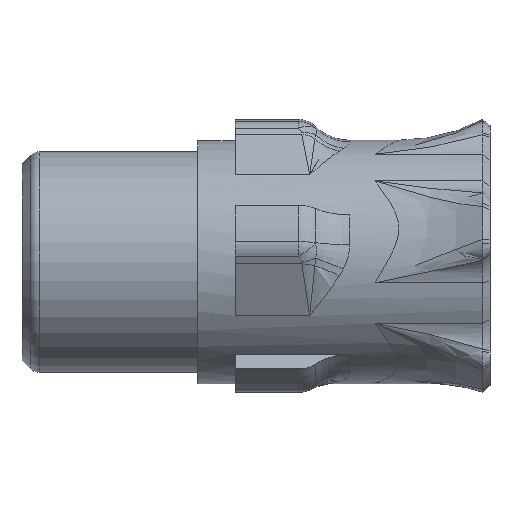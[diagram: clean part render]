
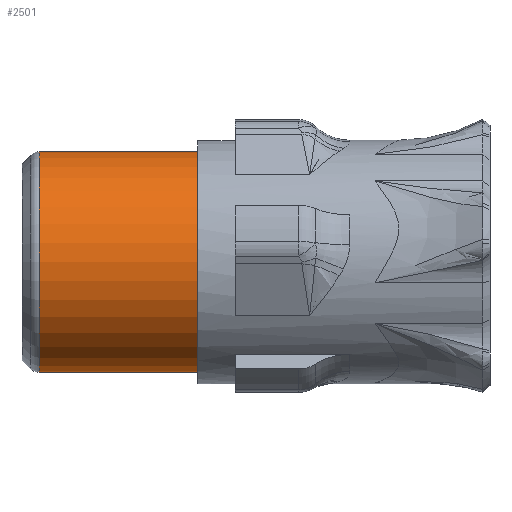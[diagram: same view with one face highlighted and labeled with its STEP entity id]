
A CAD part, left-side view. The second image highlights one B-rep face of the part: STEP entity #2501.
In plain terms, the highlighted cylindrical face has radius 4.525 mm (diameter 9.05 mm), a full revolution.
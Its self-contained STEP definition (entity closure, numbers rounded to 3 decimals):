
#309=CYLINDRICAL_SURFACE('',#2686,4.525);
#334=LINE('',#3410,#446);
#446=VECTOR('',#2901,4.525);
#577=FACE_OUTER_BOUND('',#742,.T.);
#742=EDGE_LOOP('',(#1690,#1691,#1692,#1693,#1694));
#916=CIRCLE('',#2681,4.525);
#917=CIRCLE('',#2682,4.525);
#920=CIRCLE('',#2687,4.525);
#1031=VERTEX_POINT('',#3397);
#1032=VERTEX_POINT('',#3399);
#1034=VERTEX_POINT('',#3408);
#1278=EDGE_CURVE('',#1031,#1032,#916,.T.);
#1279=EDGE_CURVE('',#1032,#1031,#917,.T.);
#1283=EDGE_CURVE('',#1034,#1034,#920,.T.);
#1284=EDGE_CURVE('',#1034,#1032,#334,.T.);
#1690=ORIENTED_EDGE('',*,*,#1283,.F.);
#1691=ORIENTED_EDGE('',*,*,#1284,.T.);
#1692=ORIENTED_EDGE('',*,*,#1278,.F.);
#1693=ORIENTED_EDGE('',*,*,#1279,.F.);
#1694=ORIENTED_EDGE('',*,*,#1284,.F.);
#2501=ADVANCED_FACE('',(#577),#309,.T.);
#2681=AXIS2_PLACEMENT_3D('',#3400,#2886,#2887);
#2682=AXIS2_PLACEMENT_3D('',#3401,#2888,#2889);
#2686=AXIS2_PLACEMENT_3D('',#3407,#2897,#2898);
#2687=AXIS2_PLACEMENT_3D('',#3409,#2899,#2900);
#2886=DIRECTION('center_axis',(0.,1.,0.));
#2887=DIRECTION('ref_axis',(1.,0.,0.));
#2888=DIRECTION('center_axis',(0.,1.,0.));
#2889=DIRECTION('ref_axis',(1.,0.,0.));
#2897=DIRECTION('center_axis',(0.,-1.,0.));
#2898=DIRECTION('ref_axis',(1.,0.,0.));
#2899=DIRECTION('center_axis',(0.,-1.,0.));
#2900=DIRECTION('ref_axis',(1.,0.,0.));
#2901=DIRECTION('',(0.,1.,0.));
#3397=CARTESIAN_POINT('',(-121.3,-23.207,-4.525));
#3399=CARTESIAN_POINT('',(-125.825,-23.207,0.));
#3400=CARTESIAN_POINT('Origin',(-121.3,-23.207,0.));
#3401=CARTESIAN_POINT('Origin',(-121.3,-23.207,0.));
#3407=CARTESIAN_POINT('Origin',(-121.3,-22.5,0.));
#3408=CARTESIAN_POINT('',(-125.825,-29.7,0.));
#3409=CARTESIAN_POINT('Origin',(-121.3,-29.7,0.));
#3410=CARTESIAN_POINT('',(-125.825,-22.5,0.));
